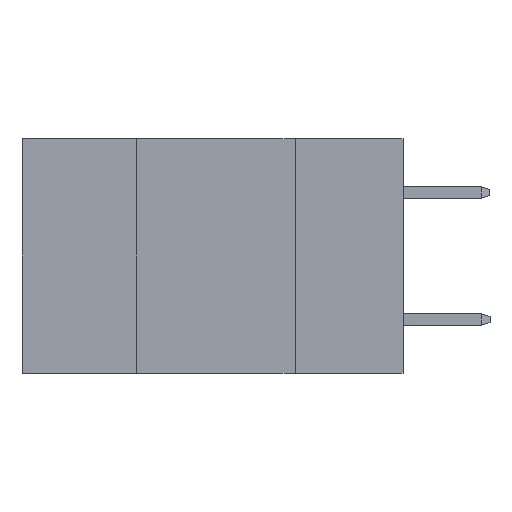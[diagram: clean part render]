
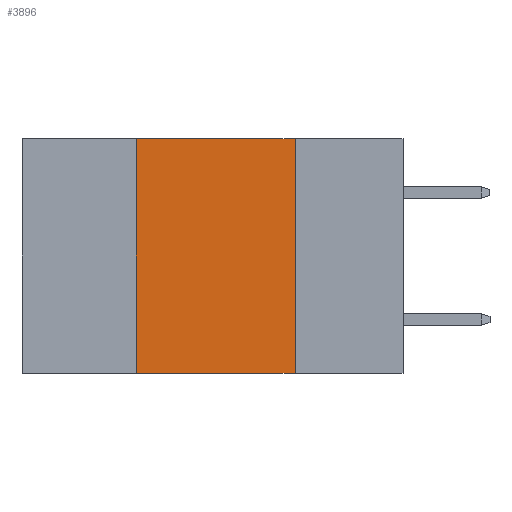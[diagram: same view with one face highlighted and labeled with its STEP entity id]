
A CAD part, left-side view. The second image highlights one B-rep face of the part: STEP entity #3896.
In plain terms, the highlighted planar face has unit normal (-1, 0, 0).
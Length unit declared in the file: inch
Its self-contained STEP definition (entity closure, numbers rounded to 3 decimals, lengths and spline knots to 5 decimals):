
#70 = LINE ( 'NONE', #3658, #10927 ) ;
#290 = VERTEX_POINT ( 'NONE', #8116 ) ;
#297 = CARTESIAN_POINT ( 'NONE',  ( 0., 0.17, 0. ) ) ;
#952 = CARTESIAN_POINT ( 'NONE',  ( 0., 0.6, 0. ) ) ;
#1072 = DIRECTION ( 'NONE',  ( 0., 0., -1. ) ) ;
#1214 = EDGE_LOOP ( 'NONE', ( #8188, #11487, #2165, #2810 ) ) ;
#1429 = CARTESIAN_POINT ( 'NONE',  ( 0., 0.6, 0. ) ) ;
#1581 = EDGE_CURVE ( 'NONE', #11472, #7672, #4523, .T. ) ;
#1630 = EDGE_CURVE ( 'NONE', #8693, #11472, #70, .T. ) ;
#1960 = DIRECTION ( 'NONE',  ( 0., 0., 1. ) ) ;
#2165 = ORIENTED_EDGE ( 'NONE', *, *, #1630, .F. ) ;
#2783 = CARTESIAN_POINT ( 'NONE',  ( 0., 0.6, -0.37 ) ) ;
#2810 = ORIENTED_EDGE ( 'NONE', *, *, #7741, .T. ) ;
#3003 = LINE ( 'NONE', #297, #3923 ) ;
#3658 = CARTESIAN_POINT ( 'NONE',  ( 0., 0.42, 0. ) ) ;
#3896 = ADVANCED_FACE ( 'NONE', ( #11173 ), #9403, .F. ) ;
#3923 = VECTOR ( 'NONE', #1072, 39.37008 ) ;
#4523 = LINE ( 'NONE', #952, #5842 ) ;
#4560 = AXIS2_PLACEMENT_3D ( 'NONE', #1429, #8468, #11405 ) ;
#4934 = CARTESIAN_POINT ( 'NONE',  ( 0., 0.42, -0.37 ) ) ;
#5738 = VECTOR ( 'NONE', #10640, 39.37008 ) ;
#5842 = VECTOR ( 'NONE', #8120, 39.37008 ) ;
#6631 = CARTESIAN_POINT ( 'NONE',  ( 0., 0.42, 0. ) ) ;
#7672 = VERTEX_POINT ( 'NONE', #8942 ) ;
#7741 = EDGE_CURVE ( 'NONE', #8693, #290, #7956, .T. ) ;
#7956 = LINE ( 'NONE', #2783, #5738 ) ;
#8116 = CARTESIAN_POINT ( 'NONE',  ( 0., 0.17, -0.37 ) ) ;
#8120 = DIRECTION ( 'NONE',  ( 0., -1., 0. ) ) ;
#8188 = ORIENTED_EDGE ( 'NONE', *, *, #10173, .F. ) ;
#8468 = DIRECTION ( 'NONE',  ( 1., 0., 0. ) ) ;
#8693 = VERTEX_POINT ( 'NONE', #4934 ) ;
#8942 = CARTESIAN_POINT ( 'NONE',  ( 0., 0.17, 0. ) ) ;
#9403 = PLANE ( 'NONE',  #4560 ) ;
#10173 = EDGE_CURVE ( 'NONE', #7672, #290, #3003, .T. ) ;
#10640 = DIRECTION ( 'NONE',  ( 0., -1., 0. ) ) ;
#10927 = VECTOR ( 'NONE', #1960, 39.37008 ) ;
#11173 = FACE_OUTER_BOUND ( 'NONE', #1214, .T. ) ;
#11405 = DIRECTION ( 'NONE',  ( 0., 0., -1. ) ) ;
#11472 = VERTEX_POINT ( 'NONE', #6631 ) ;
#11487 = ORIENTED_EDGE ( 'NONE', *, *, #1581, .F. ) ;
